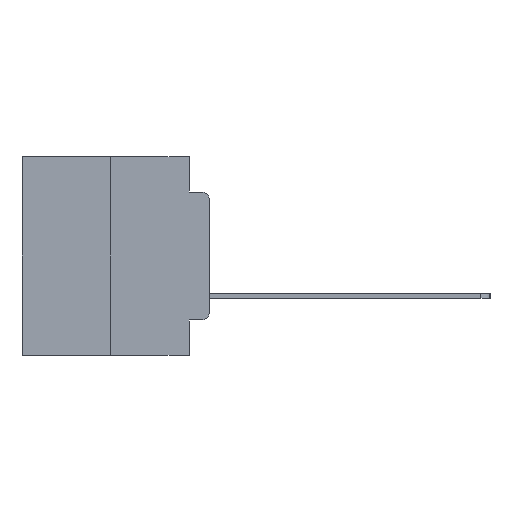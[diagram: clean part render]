
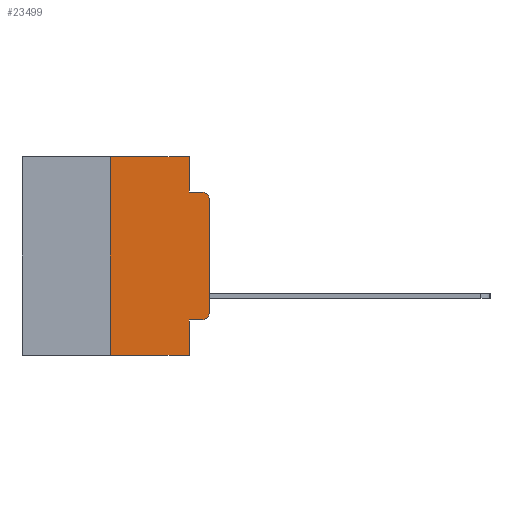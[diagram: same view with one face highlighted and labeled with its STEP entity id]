
A CAD part, left-side view. The second image highlights one B-rep face of the part: STEP entity #23499.
In plain terms, the highlighted planar face has unit normal (-1, 0, 0).
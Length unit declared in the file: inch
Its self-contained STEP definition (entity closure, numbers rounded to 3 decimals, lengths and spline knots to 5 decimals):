
#77 = EDGE_CURVE ( 'NONE', #4127, #24291, #13827, .T. ) ;
#319 = CIRCLE ( 'NONE', #3181, 0.02 ) ;
#509 = DIRECTION ( 'NONE',  ( -1., 0., 0. ) ) ;
#1125 = CARTESIAN_POINT ( 'NONE',  ( 0., 0.051, -0.0885 ) ) ;
#1337 = DIRECTION ( 'NONE',  ( 0., 0., -1. ) ) ;
#1358 = LINE ( 'NONE', #17119, #22562 ) ;
#2000 = CARTESIAN_POINT ( 'NONE',  ( 0., 0.473, 0. ) ) ;
#2523 = AXIS2_PLACEMENT_3D ( 'NONE', #13837, #2745, #18093 ) ;
#2602 = VERTEX_POINT ( 'NONE', #15948 ) ;
#2745 = DIRECTION ( 'NONE',  ( 1., 0., 0. ) ) ;
#2839 = CARTESIAN_POINT ( 'NONE',  ( 0., 0.02, -0.4115 ) ) ;
#3181 = AXIS2_PLACEMENT_3D ( 'NONE', #13856, #509, #15998 ) ;
#3351 = EDGE_CURVE ( 'NONE', #8870, #11465, #13380, .T. ) ;
#4127 = VERTEX_POINT ( 'NONE', #2839 ) ;
#4183 = ORIENTED_EDGE ( 'NONE', *, *, #3351, .F. ) ;
#4248 = CARTESIAN_POINT ( 'NONE',  ( 0., 0.25, 0. ) ) ;
#4314 = EDGE_LOOP ( 'NONE', ( #21900, #17538, #8751, #25818, #4183, #10116, #27154, #22886, #7694, #8421 ) ) ;
#4884 = LINE ( 'NONE', #1125, #27163 ) ;
#4955 = AXIS2_PLACEMENT_3D ( 'NONE', #14902, #9274, #21294 ) ;
#5665 = VERTEX_POINT ( 'NONE', #16899 ) ;
#6176 = VERTEX_POINT ( 'NONE', #7911 ) ;
#6612 = EDGE_CURVE ( 'NONE', #2602, #5665, #319, .T. ) ;
#6824 = DIRECTION ( 'NONE',  ( 0., -1., 0. ) ) ;
#7622 = VECTOR ( 'NONE', #27959, 39.37008 ) ;
#7694 = ORIENTED_EDGE ( 'NONE', *, *, #23997, .T. ) ;
#7911 = CARTESIAN_POINT ( 'NONE',  ( 0., 0.051, -0.5 ) ) ;
#8261 = VERTEX_POINT ( 'NONE', #25817 ) ;
#8343 = LINE ( 'NONE', #10926, #7622 ) ;
#8421 = ORIENTED_EDGE ( 'NONE', *, *, #77, .T. ) ;
#8447 = DIRECTION ( 'NONE',  ( 0., -1., 0. ) ) ;
#8506 = DIRECTION ( 'NONE',  ( 0., 0., 1. ) ) ;
#8751 = ORIENTED_EDGE ( 'NONE', *, *, #11119, .F. ) ;
#8870 = VERTEX_POINT ( 'NONE', #4248 ) ;
#9274 = DIRECTION ( 'NONE',  ( -1., 0., 0. ) ) ;
#9934 = CARTESIAN_POINT ( 'NONE',  ( 0., 0.25, 0. ) ) ;
#10062 = LINE ( 'NONE', #21058, #27763 ) ;
#10101 = LINE ( 'NONE', #11248, #15212 ) ;
#10116 = ORIENTED_EDGE ( 'NONE', *, *, #16879, .F. ) ;
#10410 = CARTESIAN_POINT ( 'NONE',  ( 0., 0.25, -0.5 ) ) ;
#10647 = EDGE_CURVE ( 'NONE', #26657, #6176, #16587, .T. ) ;
#10835 = CARTESIAN_POINT ( 'NONE',  ( 0., 0.051, -0.0885 ) ) ;
#10926 = CARTESIAN_POINT ( 'NONE',  ( 0., 0.051, 0. ) ) ;
#11119 = EDGE_CURVE ( 'NONE', #26159, #5665, #4884, .T. ) ;
#11248 = CARTESIAN_POINT ( 'NONE',  ( 0., 0.051, -0.4115 ) ) ;
#11300 = EDGE_CURVE ( 'NONE', #24291, #2602, #1358, .T. ) ;
#11465 = VERTEX_POINT ( 'NONE', #26086 ) ;
#12226 = VECTOR ( 'NONE', #8447, 39.37008 ) ;
#12260 = DIRECTION ( 'NONE',  ( 0., -1., 0. ) ) ;
#13380 = LINE ( 'NONE', #2000, #24654 ) ;
#13827 = CIRCLE ( 'NONE', #4955, 0.02 ) ;
#13837 = CARTESIAN_POINT ( 'NONE',  ( 0., 0.473, 0. ) ) ;
#13856 = CARTESIAN_POINT ( 'NONE',  ( 0., 0.02, -0.1085 ) ) ;
#14313 = DIRECTION ( 'NONE',  ( 0., 0., 1. ) ) ;
#14902 = CARTESIAN_POINT ( 'NONE',  ( 0., 0.02, -0.3915 ) ) ;
#15212 = VECTOR ( 'NONE', #6824, 39.37008 ) ;
#15456 = EDGE_CURVE ( 'NONE', #11465, #26159, #10062, .T. ) ;
#15948 = CARTESIAN_POINT ( 'NONE',  ( 0., 0., -0.1085 ) ) ;
#15998 = DIRECTION ( 'NONE',  ( 0., 0., -1. ) ) ;
#16587 = LINE ( 'NONE', #21370, #12226 ) ;
#16879 = EDGE_CURVE ( 'NONE', #26657, #8870, #21946, .T. ) ;
#16899 = CARTESIAN_POINT ( 'NONE',  ( 0., 0.02, -0.0885 ) ) ;
#17119 = CARTESIAN_POINT ( 'NONE',  ( 0., 0., 0. ) ) ;
#17395 = DIRECTION ( 'NONE',  ( 0., -1., 0. ) ) ;
#17538 = ORIENTED_EDGE ( 'NONE', *, *, #6612, .T. ) ;
#18093 = DIRECTION ( 'NONE',  ( 0., 0., -1. ) ) ;
#18301 = EDGE_CURVE ( 'NONE', #8261, #6176, #8343, .T. ) ;
#18713 = CARTESIAN_POINT ( 'NONE',  ( 0., 0., -0.3915 ) ) ;
#21058 = CARTESIAN_POINT ( 'NONE',  ( 0., 0.051, 0. ) ) ;
#21294 = DIRECTION ( 'NONE',  ( 0., 0., -1. ) ) ;
#21370 = CARTESIAN_POINT ( 'NONE',  ( 0., 0.473, -0.5 ) ) ;
#21900 = ORIENTED_EDGE ( 'NONE', *, *, #11300, .T. ) ;
#21946 = LINE ( 'NONE', #9934, #26850 ) ;
#22562 = VECTOR ( 'NONE', #8506, 39.37008 ) ;
#22886 = ORIENTED_EDGE ( 'NONE', *, *, #18301, .F. ) ;
#22897 = FACE_OUTER_BOUND ( 'NONE', #4314, .T. ) ;
#23499 = ADVANCED_FACE ( 'NONE', ( #22897 ), #24404, .F. ) ;
#23997 = EDGE_CURVE ( 'NONE', #8261, #4127, #10101, .T. ) ;
#24291 = VERTEX_POINT ( 'NONE', #18713 ) ;
#24404 = PLANE ( 'NONE',  #2523 ) ;
#24654 = VECTOR ( 'NONE', #17395, 39.37008 ) ;
#25817 = CARTESIAN_POINT ( 'NONE',  ( 0., 0.051, -0.4115 ) ) ;
#25818 = ORIENTED_EDGE ( 'NONE', *, *, #15456, .F. ) ;
#26086 = CARTESIAN_POINT ( 'NONE',  ( 0., 0.051, 0. ) ) ;
#26159 = VERTEX_POINT ( 'NONE', #10835 ) ;
#26657 = VERTEX_POINT ( 'NONE', #10410 ) ;
#26850 = VECTOR ( 'NONE', #14313, 39.37008 ) ;
#27154 = ORIENTED_EDGE ( 'NONE', *, *, #10647, .T. ) ;
#27163 = VECTOR ( 'NONE', #12260, 39.37008 ) ;
#27763 = VECTOR ( 'NONE', #1337, 39.37008 ) ;
#27959 = DIRECTION ( 'NONE',  ( 0., 0., -1. ) ) ;
